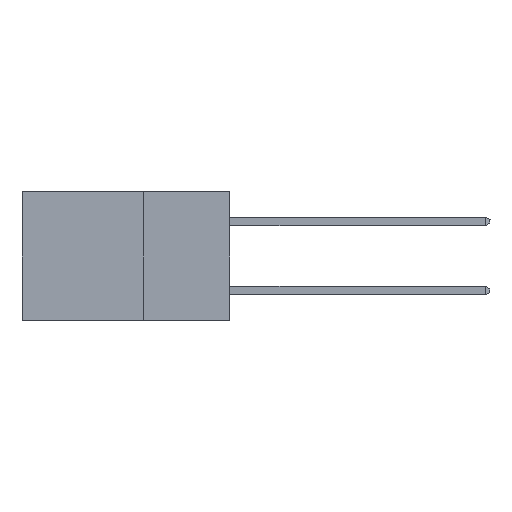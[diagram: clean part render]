
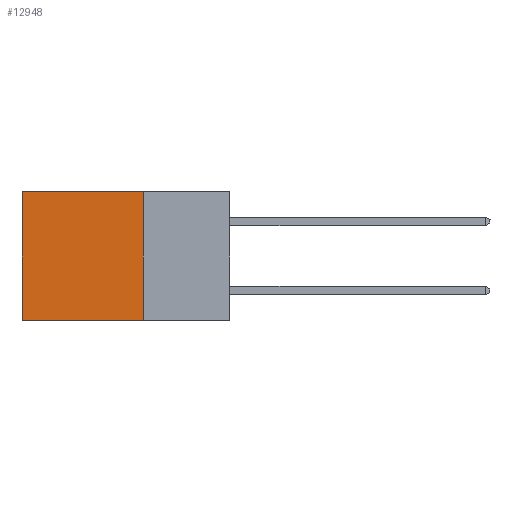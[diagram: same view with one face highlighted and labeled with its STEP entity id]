
A CAD part, left-side view. The second image highlights one B-rep face of the part: STEP entity #12948.
In plain terms, the highlighted planar face has unit normal (-1, 0, 0).
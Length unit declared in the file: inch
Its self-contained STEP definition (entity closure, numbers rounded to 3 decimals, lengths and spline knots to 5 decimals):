
#1702 = ORIENTED_EDGE ( 'NONE', *, *, #15798, .T. ) ;
#3002 = DIRECTION ( 'NONE',  ( 0., 1., 0. ) ) ;
#3724 = VERTEX_POINT ( 'NONE', #17918 ) ;
#3972 = DIRECTION ( 'NONE',  ( 1., 0., 0. ) ) ;
#4075 = CARTESIAN_POINT ( 'NONE',  ( 0.2615, 0.25, -0.37 ) ) ;
#4222 = VECTOR ( 'NONE', #6580, 39.37008 ) ;
#4666 = LINE ( 'NONE', #8597, #20776 ) ;
#5439 = LINE ( 'NONE', #7360, #15322 ) ;
#6076 = ORIENTED_EDGE ( 'NONE', *, *, #21751, .F. ) ;
#6580 = DIRECTION ( 'NONE',  ( 0., 1., 0. ) ) ;
#6703 = CARTESIAN_POINT ( 'NONE',  ( 0.2615, 0.25, -0.37 ) ) ;
#7360 = CARTESIAN_POINT ( 'NONE',  ( 0.2615, 0.25, 0. ) ) ;
#8597 = CARTESIAN_POINT ( 'NONE',  ( 0.2615, 0.25, -0.37 ) ) ;
#9387 = ORIENTED_EDGE ( 'NONE', *, *, #9943, .T. ) ;
#9860 = EDGE_LOOP ( 'NONE', ( #9387, #6076, #22122, #1702 ) ) ;
#9943 = EDGE_CURVE ( 'NONE', #11681, #3724, #10065, .T. ) ;
#10065 = LINE ( 'NONE', #18341, #22002 ) ;
#10224 = CARTESIAN_POINT ( 'NONE',  ( 0.2615, 0.25, -0.37 ) ) ;
#10788 = LINE ( 'NONE', #6703, #4222 ) ;
#11681 = VERTEX_POINT ( 'NONE', #21083 ) ;
#11840 = VERTEX_POINT ( 'NONE', #4075 ) ;
#12948 = ADVANCED_FACE ( 'NONE', ( #22575 ), #24224, .F. ) ;
#13699 = CARTESIAN_POINT ( 'NONE',  ( 0.2615, 0.25, 0. ) ) ;
#14429 = DIRECTION ( 'NONE',  ( 0., 0., -1. ) ) ;
#15322 = VECTOR ( 'NONE', #3002, 39.37008 ) ;
#15798 = EDGE_CURVE ( 'NONE', #22342, #11681, #5439, .T. ) ;
#17804 = AXIS2_PLACEMENT_3D ( 'NONE', #10224, #3972, #20534 ) ;
#17918 = CARTESIAN_POINT ( 'NONE',  ( 0.2615, 0.6, -0.37 ) ) ;
#18341 = CARTESIAN_POINT ( 'NONE',  ( 0.2615, 0.6, -0.37 ) ) ;
#20534 = DIRECTION ( 'NONE',  ( 0., 0., -1. ) ) ;
#20776 = VECTOR ( 'NONE', #14429, 39.37008 ) ;
#21083 = CARTESIAN_POINT ( 'NONE',  ( 0.2615, 0.6, 0. ) ) ;
#21751 = EDGE_CURVE ( 'NONE', #11840, #3724, #10788, .T. ) ;
#22002 = VECTOR ( 'NONE', #26654, 39.37008 ) ;
#22122 = ORIENTED_EDGE ( 'NONE', *, *, #23540, .F. ) ;
#22342 = VERTEX_POINT ( 'NONE', #13699 ) ;
#22575 = FACE_OUTER_BOUND ( 'NONE', #9860, .T. ) ;
#23540 = EDGE_CURVE ( 'NONE', #22342, #11840, #4666, .T. ) ;
#24224 = PLANE ( 'NONE',  #17804 ) ;
#26654 = DIRECTION ( 'NONE',  ( 0., 0., -1. ) ) ;
